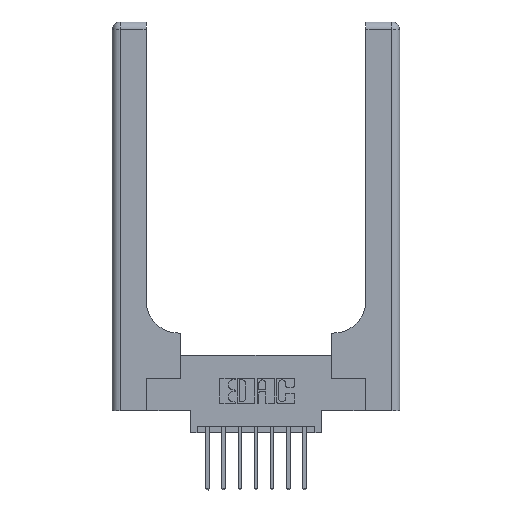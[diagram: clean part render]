
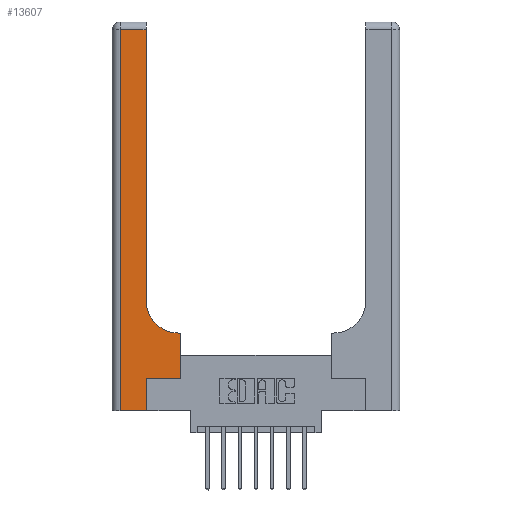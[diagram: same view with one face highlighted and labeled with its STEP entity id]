
A CAD part, top view. The second image highlights one B-rep face of the part: STEP entity #13607.
In plain terms, the highlighted planar face has unit normal (0, 0, 1).
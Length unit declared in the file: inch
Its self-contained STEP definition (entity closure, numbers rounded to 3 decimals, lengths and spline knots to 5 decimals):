
#362 = CARTESIAN_POINT ( 'NONE',  ( 0., 2.94, 0.37 ) ) ;
#478 = ORIENTED_EDGE ( 'NONE', *, *, #4250, .T. ) ;
#642 = VECTOR ( 'NONE', #5450, 39.37008 ) ;
#929 = VERTEX_POINT ( 'NONE', #2771 ) ;
#998 = EDGE_CURVE ( 'NONE', #13846, #1910, #4046, .T. ) ;
#1352 = ORIENTED_EDGE ( 'NONE', *, *, #6947, .T. ) ;
#1508 = DIRECTION ( 'NONE',  ( -1., 0., 0. ) ) ;
#1539 = ORIENTED_EDGE ( 'NONE', *, *, #7855, .T. ) ;
#1683 = ORIENTED_EDGE ( 'NONE', *, *, #12834, .T. ) ;
#1724 = ORIENTED_EDGE ( 'NONE', *, *, #2836, .T. ) ;
#1910 = VERTEX_POINT ( 'NONE', #1994 ) ;
#1994 = CARTESIAN_POINT ( 'NONE',  ( 0.528, 0.6, 0.37 ) ) ;
#2016 = FACE_OUTER_BOUND ( 'NONE', #5462, .T. ) ;
#2058 = VECTOR ( 'NONE', #10483, 39.37008 ) ;
#2155 = CARTESIAN_POINT ( 'NONE',  ( 0., 3., 0.37 ) ) ;
#2771 = CARTESIAN_POINT ( 'NONE',  ( 0.265, 0.25, 0.37 ) ) ;
#2836 = EDGE_CURVE ( 'NONE', #3149, #14640, #11793, .T. ) ;
#2893 = DIRECTION ( 'NONE',  ( 0., 0., -1. ) ) ;
#3149 = VERTEX_POINT ( 'NONE', #11111 ) ;
#3535 = CARTESIAN_POINT ( 'NONE',  ( 0.265, 0.25, 0.37 ) ) ;
#3583 = CARTESIAN_POINT ( 'NONE',  ( 0.06, 3., 0.37 ) ) ;
#3665 = VECTOR ( 'NONE', #11523, 39.37008 ) ;
#3885 = ORIENTED_EDGE ( 'NONE', *, *, #12184, .T. ) ;
#4045 = CARTESIAN_POINT ( 'NONE',  ( 0.265, 0., 0.37 ) ) ;
#4046 = LINE ( 'NONE', #11774, #3665 ) ;
#4056 = CARTESIAN_POINT ( 'NONE',  ( 0.528, 0.25, 0.37 ) ) ;
#4250 = EDGE_CURVE ( 'NONE', #9288, #929, #4492, .T. ) ;
#4261 = ORIENTED_EDGE ( 'NONE', *, *, #5393, .T. ) ;
#4309 = VECTOR ( 'NONE', #13270, 39.37008 ) ;
#4492 = LINE ( 'NONE', #9110, #10200 ) ;
#4513 = PLANE ( 'NONE',  #10974 ) ;
#5230 = ORIENTED_EDGE ( 'NONE', *, *, #10469, .T. ) ;
#5359 = DIRECTION ( 'NONE',  ( -1., 0., 0. ) ) ;
#5393 = EDGE_CURVE ( 'NONE', #12220, #3149, #12419, .T. ) ;
#5450 = DIRECTION ( 'NONE',  ( 0., 1., 0. ) ) ;
#5462 = EDGE_LOOP ( 'NONE', ( #4261, #1724, #3885, #5230, #478, #1352, #5596, #1539, #1683 ) ) ;
#5513 = AXIS2_PLACEMENT_3D ( 'NONE', #9788, #2893, #10885 ) ;
#5596 = ORIENTED_EDGE ( 'NONE', *, *, #998, .T. ) ;
#5712 = DIRECTION ( 'NONE',  ( -1., 0., 0. ) ) ;
#6060 = CIRCLE ( 'NONE', #5513, 0.25 ) ;
#6186 = CARTESIAN_POINT ( 'NONE',  ( 0.26, 0.85, 0.37 ) ) ;
#6352 = VECTOR ( 'NONE', #5359, 39.37008 ) ;
#6641 = VERTEX_POINT ( 'NONE', #12451 ) ;
#6766 = LINE ( 'NONE', #3535, #9419 ) ;
#6947 = EDGE_CURVE ( 'NONE', #929, #13846, #6766, .T. ) ;
#7151 = CARTESIAN_POINT ( 'NONE',  ( 0.06, 2.94, 0.37 ) ) ;
#7741 = LINE ( 'NONE', #9961, #4309 ) ;
#7855 = EDGE_CURVE ( 'NONE', #1910, #6641, #9359, .T. ) ;
#8836 = VECTOR ( 'NONE', #1508, 39.37008 ) ;
#9110 = CARTESIAN_POINT ( 'NONE',  ( 0.265, 0., 0.37 ) ) ;
#9258 = DIRECTION ( 'NONE',  ( 1., 0., 0. ) ) ;
#9288 = VERTEX_POINT ( 'NONE', #4045 ) ;
#9359 = LINE ( 'NONE', #10953, #6352 ) ;
#9419 = VECTOR ( 'NONE', #9258, 39.37008 ) ;
#9684 = CARTESIAN_POINT ( 'NONE',  ( 0.06, 0., 0.37 ) ) ;
#9788 = CARTESIAN_POINT ( 'NONE',  ( 0.51, 0.85, 0.37 ) ) ;
#9961 = CARTESIAN_POINT ( 'NONE',  ( 0., 0., 0.37 ) ) ;
#10200 = VECTOR ( 'NONE', #14568, 39.37008 ) ;
#10469 = EDGE_CURVE ( 'NONE', #11418, #9288, #7741, .T. ) ;
#10483 = DIRECTION ( 'NONE',  ( 0., -1., 0. ) ) ;
#10885 = DIRECTION ( 'NONE',  ( 1., 0., 0. ) ) ;
#10953 = CARTESIAN_POINT ( 'NONE',  ( 0.26, 0.6, 0.37 ) ) ;
#10974 = AXIS2_PLACEMENT_3D ( 'NONE', #2155, #12417, #5712 ) ;
#10994 = CARTESIAN_POINT ( 'NONE',  ( 0.26, 3., 0.37 ) ) ;
#11111 = CARTESIAN_POINT ( 'NONE',  ( 0.26, 2.94, 0.37 ) ) ;
#11418 = VERTEX_POINT ( 'NONE', #9684 ) ;
#11523 = DIRECTION ( 'NONE',  ( 0., 1., 0. ) ) ;
#11774 = CARTESIAN_POINT ( 'NONE',  ( 0.528, 0.25, 0.37 ) ) ;
#11793 = LINE ( 'NONE', #362, #8836 ) ;
#12184 = EDGE_CURVE ( 'NONE', #14640, #11418, #14063, .T. ) ;
#12220 = VERTEX_POINT ( 'NONE', #6186 ) ;
#12417 = DIRECTION ( 'NONE',  ( 0., 0., -1. ) ) ;
#12419 = LINE ( 'NONE', #10994, #642 ) ;
#12451 = CARTESIAN_POINT ( 'NONE',  ( 0.51, 0.6, 0.37 ) ) ;
#12834 = EDGE_CURVE ( 'NONE', #6641, #12220, #6060, .T. ) ;
#13270 = DIRECTION ( 'NONE',  ( 1., 0., 0. ) ) ;
#13607 = ADVANCED_FACE ( 'NONE', ( #2016 ), #4513, .F. ) ;
#13846 = VERTEX_POINT ( 'NONE', #4056 ) ;
#14063 = LINE ( 'NONE', #3583, #2058 ) ;
#14568 = DIRECTION ( 'NONE',  ( 0., 1., 0. ) ) ;
#14640 = VERTEX_POINT ( 'NONE', #7151 ) ;
